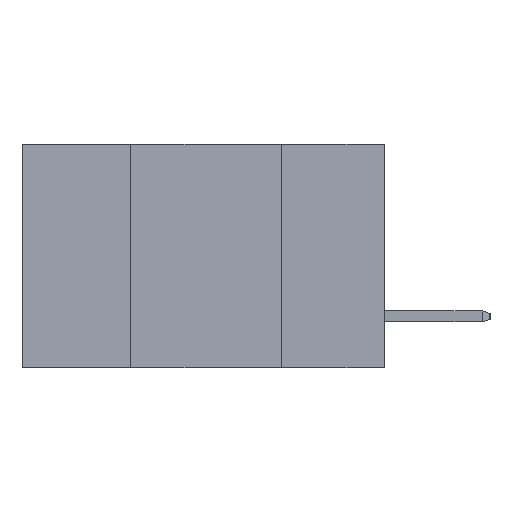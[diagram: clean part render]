
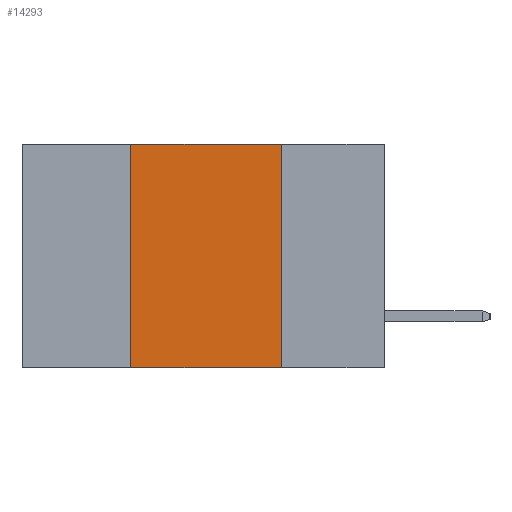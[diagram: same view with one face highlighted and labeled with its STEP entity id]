
A CAD part, left-side view. The second image highlights one B-rep face of the part: STEP entity #14293.
In plain terms, the highlighted planar face has unit normal (-1, 0, 0).
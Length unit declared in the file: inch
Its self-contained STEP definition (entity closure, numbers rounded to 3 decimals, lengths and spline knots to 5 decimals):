
#173 = CARTESIAN_POINT ( 'NONE',  ( 0., 0.42, 0. ) ) ;
#446 = CARTESIAN_POINT ( 'NONE',  ( 0., 0.42, 0. ) ) ;
#1211 = VERTEX_POINT ( 'NONE', #5197 ) ;
#1676 = LINE ( 'NONE', #173, #6583 ) ;
#3208 = DIRECTION ( 'NONE',  ( 1., 0., 0. ) ) ;
#3367 = VERTEX_POINT ( 'NONE', #5578 ) ;
#4314 = CARTESIAN_POINT ( 'NONE',  ( 0., 0.17, -0.37 ) ) ;
#4934 = AXIS2_PLACEMENT_3D ( 'NONE', #6366, #3208, #14645 ) ;
#5197 = CARTESIAN_POINT ( 'NONE',  ( 0., 0.42, -0.37 ) ) ;
#5353 = VECTOR ( 'NONE', #10068, 39.37008 ) ;
#5578 = CARTESIAN_POINT ( 'NONE',  ( 0., 0.17, 0. ) ) ;
#5858 = LINE ( 'NONE', #8441, #5353 ) ;
#6366 = CARTESIAN_POINT ( 'NONE',  ( 0., 0.6, 0. ) ) ;
#6583 = VECTOR ( 'NONE', #11669, 39.37008 ) ;
#7103 = ORIENTED_EDGE ( 'NONE', *, *, #14736, .T. ) ;
#7660 = DIRECTION ( 'NONE',  ( 0., 0., -1. ) ) ;
#8345 = EDGE_CURVE ( 'NONE', #3367, #12534, #9088, .T. ) ;
#8441 = CARTESIAN_POINT ( 'NONE',  ( 0., 0.6, 0. ) ) ;
#9088 = LINE ( 'NONE', #15735, #17130 ) ;
#9178 = DIRECTION ( 'NONE',  ( 0., -1., 0. ) ) ;
#9769 = PLANE ( 'NONE',  #4934 ) ;
#10068 = DIRECTION ( 'NONE',  ( 0., -1., 0. ) ) ;
#10389 = FACE_OUTER_BOUND ( 'NONE', #18561, .T. ) ;
#10442 = ORIENTED_EDGE ( 'NONE', *, *, #18208, .F. ) ;
#11669 = DIRECTION ( 'NONE',  ( 0., 0., 1. ) ) ;
#12232 = EDGE_CURVE ( 'NONE', #1211, #16990, #1676, .T. ) ;
#12534 = VERTEX_POINT ( 'NONE', #4314 ) ;
#14293 = ADVANCED_FACE ( 'NONE', ( #10389 ), #9769, .F. ) ;
#14457 = VECTOR ( 'NONE', #9178, 39.37008 ) ;
#14645 = DIRECTION ( 'NONE',  ( 0., 0., -1. ) ) ;
#14736 = EDGE_CURVE ( 'NONE', #1211, #12534, #18671, .T. ) ;
#15231 = ORIENTED_EDGE ( 'NONE', *, *, #12232, .F. ) ;
#15735 = CARTESIAN_POINT ( 'NONE',  ( 0., 0.17, 0. ) ) ;
#16990 = VERTEX_POINT ( 'NONE', #446 ) ;
#17130 = VECTOR ( 'NONE', #7660, 39.37008 ) ;
#17196 = CARTESIAN_POINT ( 'NONE',  ( 0., 0.6, -0.37 ) ) ;
#18208 = EDGE_CURVE ( 'NONE', #16990, #3367, #5858, .T. ) ;
#18460 = ORIENTED_EDGE ( 'NONE', *, *, #8345, .F. ) ;
#18561 = EDGE_LOOP ( 'NONE', ( #18460, #10442, #15231, #7103 ) ) ;
#18671 = LINE ( 'NONE', #17196, #14457 ) ;
